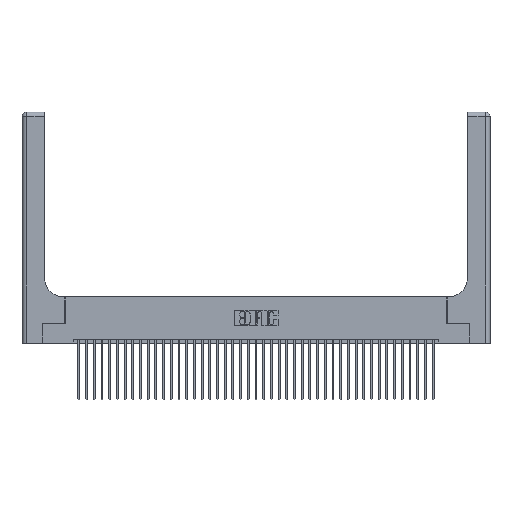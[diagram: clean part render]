
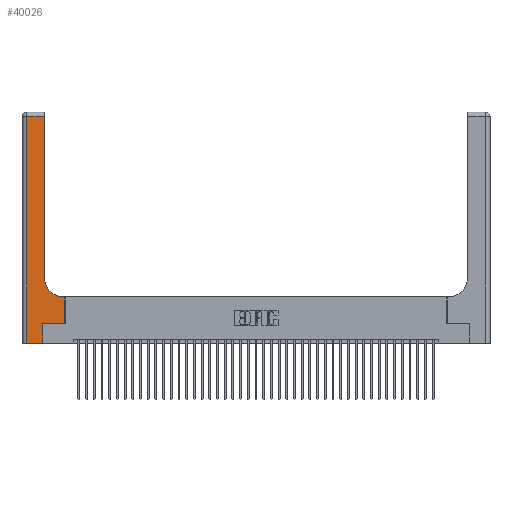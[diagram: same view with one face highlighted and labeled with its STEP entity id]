
A CAD part, top view. The second image highlights one B-rep face of the part: STEP entity #40026.
In plain terms, the highlighted planar face has unit normal (0, 0, 1).
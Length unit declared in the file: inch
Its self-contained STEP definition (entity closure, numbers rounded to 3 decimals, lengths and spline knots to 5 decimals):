
#568 = CARTESIAN_POINT ( 'NONE',  ( 0.5585, 0.25, 0.37 ) ) ;
#634 = ORIENTED_EDGE ( 'NONE', *, *, #35938, .T. ) ;
#653 = CIRCLE ( 'NONE', #5117, 0.25 ) ;
#970 = CARTESIAN_POINT ( 'NONE',  ( 0.5585, 0.6, 0.37 ) ) ;
#1220 = EDGE_CURVE ( 'NONE', #27208, #18281, #38286, .T. ) ;
#1895 = EDGE_CURVE ( 'NONE', #34342, #19685, #653, .T. ) ;
#2631 = DIRECTION ( 'NONE',  ( 0., 1., 0. ) ) ;
#2983 = DIRECTION ( 'NONE',  ( 1., 0., 0. ) ) ;
#3061 = CARTESIAN_POINT ( 'NONE',  ( 0.269, 0., 0.37 ) ) ;
#3626 = DIRECTION ( 'NONE',  ( 0., 0., -1. ) ) ;
#3773 = CARTESIAN_POINT ( 'NONE',  ( 0.5585, 0.25, 0.37 ) ) ;
#4151 = DIRECTION ( 'NONE',  ( -1., 0., 0. ) ) ;
#5117 = AXIS2_PLACEMENT_3D ( 'NONE', #35228, #15709, #28507 ) ;
#6119 = VECTOR ( 'NONE', #38700, 39.37008 ) ;
#6331 = ORIENTED_EDGE ( 'NONE', *, *, #7990, .T. ) ;
#7870 = DIRECTION ( 'NONE',  ( 0., -1., 0. ) ) ;
#7953 = ORIENTED_EDGE ( 'NONE', *, *, #1220, .T. ) ;
#7990 = EDGE_CURVE ( 'NONE', #29528, #27208, #10757, .T. ) ;
#9077 = CARTESIAN_POINT ( 'NONE',  ( 0.2915, 0.6, 0.37 ) ) ;
#10726 = LINE ( 'NONE', #25684, #13737 ) ;
#10757 = LINE ( 'NONE', #15462, #41362 ) ;
#11835 = ORIENTED_EDGE ( 'NONE', *, *, #1895, .T. ) ;
#11983 = ORIENTED_EDGE ( 'NONE', *, *, #37066, .T. ) ;
#13737 = VECTOR ( 'NONE', #22635, 39.37008 ) ;
#14189 = ORIENTED_EDGE ( 'NONE', *, *, #31991, .T. ) ;
#15125 = LINE ( 'NONE', #3773, #6119 ) ;
#15462 = CARTESIAN_POINT ( 'NONE',  ( 0., 0., 0.37 ) ) ;
#15707 = VECTOR ( 'NONE', #18870, 39.37008 ) ;
#15709 = DIRECTION ( 'NONE',  ( 0., 0., -1. ) ) ;
#16876 = CARTESIAN_POINT ( 'NONE',  ( 0., 3., 0.37 ) ) ;
#17311 = LINE ( 'NONE', #20231, #31835 ) ;
#18010 = FACE_OUTER_BOUND ( 'NONE', #26537, .T. ) ;
#18281 = VERTEX_POINT ( 'NONE', #25603 ) ;
#18870 = DIRECTION ( 'NONE',  ( -1., 0., 0. ) ) ;
#19389 = CARTESIAN_POINT ( 'NONE',  ( 0.2915, 0.85, 0.37 ) ) ;
#19685 = VERTEX_POINT ( 'NONE', #19389 ) ;
#19927 = PLANE ( 'NONE',  #26672 ) ;
#20231 = CARTESIAN_POINT ( 'NONE',  ( 0., 2.94, 0.37 ) ) ;
#20639 = ORIENTED_EDGE ( 'NONE', *, *, #30715, .T. ) ;
#20988 = CARTESIAN_POINT ( 'NONE',  ( 0.2915, 2.94, 0.37 ) ) ;
#22635 = DIRECTION ( 'NONE',  ( 0., 1., 0. ) ) ;
#23016 = VECTOR ( 'NONE', #2983, 39.37008 ) ;
#23871 = VERTEX_POINT ( 'NONE', #970 ) ;
#23998 = VERTEX_POINT ( 'NONE', #20988 ) ;
#24730 = VECTOR ( 'NONE', #2631, 39.37008 ) ;
#24763 = CARTESIAN_POINT ( 'NONE',  ( 0.06, 0., 0.37 ) ) ;
#24911 = DIRECTION ( 'NONE',  ( 1., 0., 0. ) ) ;
#25603 = CARTESIAN_POINT ( 'NONE',  ( 0.269, 0.25, 0.37 ) ) ;
#25684 = CARTESIAN_POINT ( 'NONE',  ( 0.2915, 3., 0.37 ) ) ;
#26198 = DIRECTION ( 'NONE',  ( -1., 0., 0. ) ) ;
#26537 = EDGE_LOOP ( 'NONE', ( #11983, #634, #14189, #6331, #7953, #29473, #33677, #20639, #11835 ) ) ;
#26672 = AXIS2_PLACEMENT_3D ( 'NONE', #16876, #3626, #4151 ) ;
#27070 = VECTOR ( 'NONE', #7870, 39.37008 ) ;
#27089 = VERTEX_POINT ( 'NONE', #30736 ) ;
#27208 = VERTEX_POINT ( 'NONE', #41170 ) ;
#28278 = EDGE_CURVE ( 'NONE', #18281, #36627, #34526, .T. ) ;
#28434 = CARTESIAN_POINT ( 'NONE',  ( 0.5415, 0.6, 0.37 ) ) ;
#28507 = DIRECTION ( 'NONE',  ( 1., 0., 0. ) ) ;
#29473 = ORIENTED_EDGE ( 'NONE', *, *, #28278, .T. ) ;
#29528 = VERTEX_POINT ( 'NONE', #24763 ) ;
#30715 = EDGE_CURVE ( 'NONE', #23871, #34342, #38217, .T. ) ;
#30736 = CARTESIAN_POINT ( 'NONE',  ( 0.06, 2.94, 0.37 ) ) ;
#31835 = VECTOR ( 'NONE', #26198, 39.37008 ) ;
#31991 = EDGE_CURVE ( 'NONE', #27089, #29528, #34605, .T. ) ;
#33677 = ORIENTED_EDGE ( 'NONE', *, *, #39048, .T. ) ;
#34342 = VERTEX_POINT ( 'NONE', #28434 ) ;
#34526 = LINE ( 'NONE', #34926, #23016 ) ;
#34605 = LINE ( 'NONE', #40037, #27070 ) ;
#34926 = CARTESIAN_POINT ( 'NONE',  ( 0.269, 0.25, 0.37 ) ) ;
#35228 = CARTESIAN_POINT ( 'NONE',  ( 0.5415, 0.85, 0.37 ) ) ;
#35938 = EDGE_CURVE ( 'NONE', #23998, #27089, #17311, .T. ) ;
#36627 = VERTEX_POINT ( 'NONE', #568 ) ;
#37066 = EDGE_CURVE ( 'NONE', #19685, #23998, #10726, .T. ) ;
#38217 = LINE ( 'NONE', #9077, #15707 ) ;
#38286 = LINE ( 'NONE', #3061, #24730 ) ;
#38700 = DIRECTION ( 'NONE',  ( 0., 1., 0. ) ) ;
#39048 = EDGE_CURVE ( 'NONE', #36627, #23871, #15125, .T. ) ;
#40026 = ADVANCED_FACE ( 'NONE', ( #18010 ), #19927, .F. ) ;
#40037 = CARTESIAN_POINT ( 'NONE',  ( 0.06, 3., 0.37 ) ) ;
#41170 = CARTESIAN_POINT ( 'NONE',  ( 0.269, 0., 0.37 ) ) ;
#41362 = VECTOR ( 'NONE', #24911, 39.37008 ) ;
